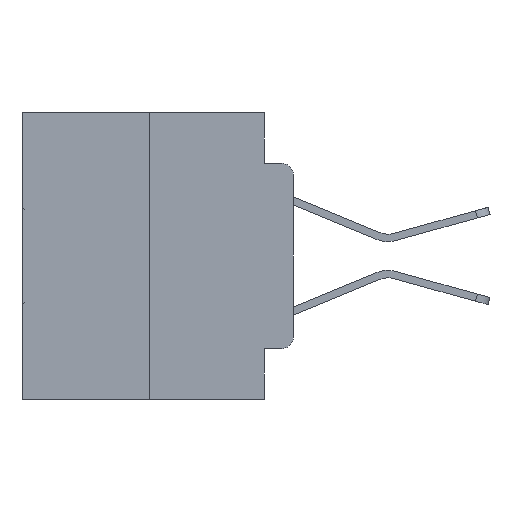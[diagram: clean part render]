
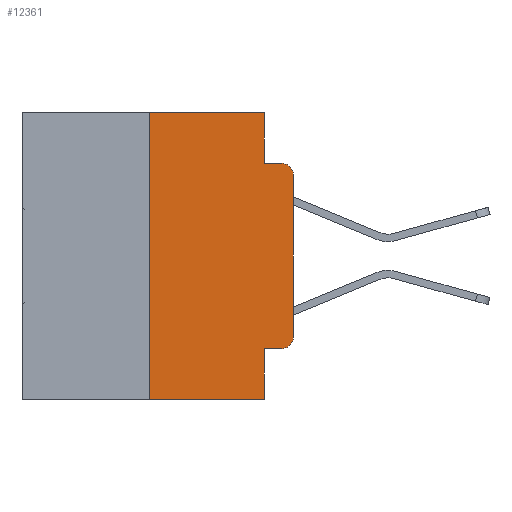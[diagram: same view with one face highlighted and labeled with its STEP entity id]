
A CAD part, left-side view. The second image highlights one B-rep face of the part: STEP entity #12361.
In plain terms, the highlighted planar face has unit normal (-1, 0, 0).
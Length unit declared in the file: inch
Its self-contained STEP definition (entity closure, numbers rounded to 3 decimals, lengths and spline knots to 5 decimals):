
#371 = CARTESIAN_POINT ( 'NONE',  ( 0., 0.051, 0. ) ) ;
#412 = DIRECTION ( 'NONE',  ( 0., 0., 1. ) ) ;
#634 = VECTOR ( 'NONE', #24583, 39.37008 ) ;
#1066 = DIRECTION ( 'NONE',  ( 0., -1., 0. ) ) ;
#2063 = VERTEX_POINT ( 'NONE', #14744 ) ;
#2271 = DIRECTION ( 'NONE',  ( -1., 0., 0. ) ) ;
#3339 = CARTESIAN_POINT ( 'NONE',  ( 0., 0.473, -0.5 ) ) ;
#4003 = LINE ( 'NONE', #25382, #21779 ) ;
#4205 = CARTESIAN_POINT ( 'NONE',  ( 0., 0.051, 0. ) ) ;
#4215 = EDGE_CURVE ( 'NONE', #8875, #24738, #28400, .T. ) ;
#4434 = CARTESIAN_POINT ( 'NONE',  ( 0., 0., -0.1085 ) ) ;
#4835 = FACE_OUTER_BOUND ( 'NONE', #18022, .T. ) ;
#5317 = DIRECTION ( 'NONE',  ( 0., -1., 0. ) ) ;
#5818 = EDGE_CURVE ( 'NONE', #21978, #24738, #13026, .T. ) ;
#6307 = VERTEX_POINT ( 'NONE', #19098 ) ;
#6489 = VECTOR ( 'NONE', #5317, 39.37008 ) ;
#6597 = VERTEX_POINT ( 'NONE', #15595 ) ;
#7007 = CARTESIAN_POINT ( 'NONE',  ( 0., 0.051, -0.4115 ) ) ;
#7360 = EDGE_CURVE ( 'NONE', #17608, #21978, #11836, .T. ) ;
#7431 = AXIS2_PLACEMENT_3D ( 'NONE', #16311, #2271, #18599 ) ;
#8875 = VERTEX_POINT ( 'NONE', #23053 ) ;
#9142 = DIRECTION ( 'NONE',  ( 0., 0., -1. ) ) ;
#9430 = DIRECTION ( 'NONE',  ( 0., 0., 1. ) ) ;
#9522 = CARTESIAN_POINT ( 'NONE',  ( 0., 0., 0. ) ) ;
#9567 = DIRECTION ( 'NONE',  ( 0., 0., -1. ) ) ;
#9779 = CARTESIAN_POINT ( 'NONE',  ( 0., 0.02, -0.0885 ) ) ;
#9889 = CARTESIAN_POINT ( 'NONE',  ( 0., 0.25, 0. ) ) ;
#9996 = VECTOR ( 'NONE', #1066, 39.37008 ) ;
#11836 = LINE ( 'NONE', #9522, #23390 ) ;
#12306 = CARTESIAN_POINT ( 'NONE',  ( 0., 0.02, -0.3915 ) ) ;
#12361 = ADVANCED_FACE ( 'NONE', ( #4835 ), #16494, .F. ) ;
#12595 = VERTEX_POINT ( 'NONE', #21885 ) ;
#12843 = VECTOR ( 'NONE', #26009, 39.37008 ) ;
#13026 = CIRCLE ( 'NONE', #7431, 0.02 ) ;
#13201 = LINE ( 'NONE', #22268, #634 ) ;
#14663 = DIRECTION ( 'NONE',  ( 0., 0., -1. ) ) ;
#14744 = CARTESIAN_POINT ( 'NONE',  ( 0., 0.25, 0. ) ) ;
#15595 = CARTESIAN_POINT ( 'NONE',  ( 0., 0.051, -0.5 ) ) ;
#16006 = VERTEX_POINT ( 'NONE', #7007 ) ;
#16311 = CARTESIAN_POINT ( 'NONE',  ( 0., 0.02, -0.1085 ) ) ;
#16494 = PLANE ( 'NONE',  #19592 ) ;
#17270 = EDGE_CURVE ( 'NONE', #6307, #17608, #19740, .T. ) ;
#17608 = VERTEX_POINT ( 'NONE', #27899 ) ;
#18022 = EDGE_LOOP ( 'NONE', ( #22487, #21656, #21433, #23851, #25636, #24974, #25392, #24774, #22519, #22750 ) ) ;
#18277 = VECTOR ( 'NONE', #21915, 39.37008 ) ;
#18599 = DIRECTION ( 'NONE',  ( 0., 0., -1. ) ) ;
#19098 = CARTESIAN_POINT ( 'NONE',  ( 0., 0.02, -0.4115 ) ) ;
#19106 = CARTESIAN_POINT ( 'NONE',  ( 0., 0.051, -0.4115 ) ) ;
#19592 = AXIS2_PLACEMENT_3D ( 'NONE', #21088, #23401, #9567 ) ;
#19737 = LINE ( 'NONE', #371, #12843 ) ;
#19740 = CIRCLE ( 'NONE', #29402, 0.02 ) ;
#20247 = LINE ( 'NONE', #19106, #6489 ) ;
#20343 = EDGE_CURVE ( 'NONE', #16006, #6307, #20247, .T. ) ;
#21088 = CARTESIAN_POINT ( 'NONE',  ( 0., 0.473, 0. ) ) ;
#21433 = ORIENTED_EDGE ( 'NONE', *, *, #4215, .F. ) ;
#21656 = ORIENTED_EDGE ( 'NONE', *, *, #5818, .T. ) ;
#21779 = VECTOR ( 'NONE', #9142, 39.37008 ) ;
#21885 = CARTESIAN_POINT ( 'NONE',  ( 0., 0.25, -0.5 ) ) ;
#21915 = DIRECTION ( 'NONE',  ( 0., -1., 0. ) ) ;
#21978 = VERTEX_POINT ( 'NONE', #4434 ) ;
#21988 = VECTOR ( 'NONE', #412, 39.37008 ) ;
#22268 = CARTESIAN_POINT ( 'NONE',  ( 0., 0.473, 0. ) ) ;
#22487 = ORIENTED_EDGE ( 'NONE', *, *, #7360, .T. ) ;
#22519 = ORIENTED_EDGE ( 'NONE', *, *, #20343, .T. ) ;
#22575 = VERTEX_POINT ( 'NONE', #4205 ) ;
#22750 = ORIENTED_EDGE ( 'NONE', *, *, #17270, .T. ) ;
#23053 = CARTESIAN_POINT ( 'NONE',  ( 0., 0.051, -0.0885 ) ) ;
#23390 = VECTOR ( 'NONE', #9430, 39.37008 ) ;
#23401 = DIRECTION ( 'NONE',  ( 1., 0., 0. ) ) ;
#23420 = EDGE_CURVE ( 'NONE', #16006, #6597, #4003, .T. ) ;
#23663 = LINE ( 'NONE', #3339, #18277 ) ;
#23851 = ORIENTED_EDGE ( 'NONE', *, *, #29553, .F. ) ;
#24583 = DIRECTION ( 'NONE',  ( 0., -1., 0. ) ) ;
#24738 = VERTEX_POINT ( 'NONE', #9779 ) ;
#24774 = ORIENTED_EDGE ( 'NONE', *, *, #23420, .F. ) ;
#24974 = ORIENTED_EDGE ( 'NONE', *, *, #26528, .F. ) ;
#25382 = CARTESIAN_POINT ( 'NONE',  ( 0., 0.051, 0. ) ) ;
#25392 = ORIENTED_EDGE ( 'NONE', *, *, #28442, .T. ) ;
#25636 = ORIENTED_EDGE ( 'NONE', *, *, #29759, .F. ) ;
#26009 = DIRECTION ( 'NONE',  ( 0., 0., -1. ) ) ;
#26528 = EDGE_CURVE ( 'NONE', #12595, #2063, #28107, .T. ) ;
#27899 = CARTESIAN_POINT ( 'NONE',  ( 0., 0., -0.3915 ) ) ;
#28107 = LINE ( 'NONE', #9889, #21988 ) ;
#28400 = LINE ( 'NONE', #28917, #9996 ) ;
#28428 = DIRECTION ( 'NONE',  ( -1., 0., 0. ) ) ;
#28442 = EDGE_CURVE ( 'NONE', #12595, #6597, #23663, .T. ) ;
#28917 = CARTESIAN_POINT ( 'NONE',  ( 0., 0.051, -0.0885 ) ) ;
#29402 = AXIS2_PLACEMENT_3D ( 'NONE', #12306, #28428, #14663 ) ;
#29553 = EDGE_CURVE ( 'NONE', #22575, #8875, #19737, .T. ) ;
#29759 = EDGE_CURVE ( 'NONE', #2063, #22575, #13201, .T. ) ;
